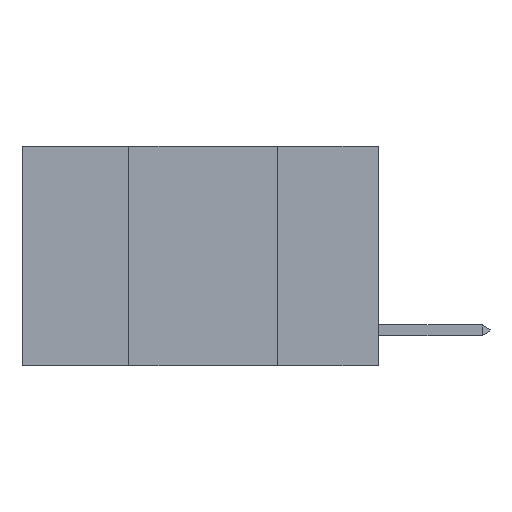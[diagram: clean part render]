
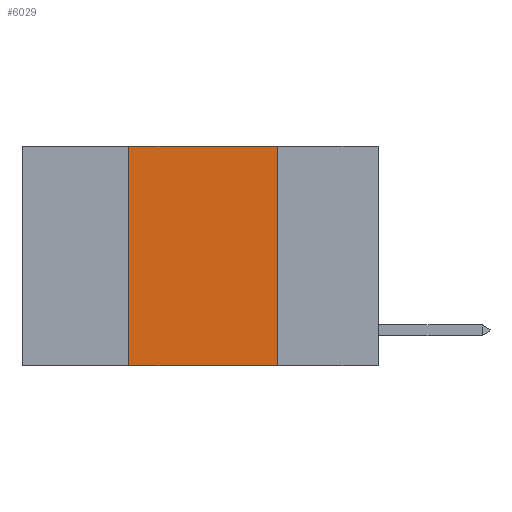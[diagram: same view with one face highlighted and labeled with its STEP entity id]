
A CAD part, left-side view. The second image highlights one B-rep face of the part: STEP entity #6029.
In plain terms, the highlighted planar face has unit normal (-1, 0, 0).
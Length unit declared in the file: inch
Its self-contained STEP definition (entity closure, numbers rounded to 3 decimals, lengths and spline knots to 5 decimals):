
#338 = CARTESIAN_POINT ( 'NONE',  ( 0., 0.6, 0. ) ) ;
#561 = EDGE_CURVE ( 'NONE', #802, #601, #5431, .T. ) ;
#601 = VERTEX_POINT ( 'NONE', #6798 ) ;
#706 = CARTESIAN_POINT ( 'NONE',  ( 0., 0.17, 0. ) ) ;
#802 = VERTEX_POINT ( 'NONE', #706 ) ;
#903 = DIRECTION ( 'NONE',  ( 0., -1., 0. ) ) ;
#1190 = ORIENTED_EDGE ( 'NONE', *, *, #10786, .F. ) ;
#1215 = VECTOR ( 'NONE', #3394, 39.37008 ) ;
#1487 = ORIENTED_EDGE ( 'NONE', *, *, #1878, .F. ) ;
#1836 = DIRECTION ( 'NONE',  ( 0., -1., 0. ) ) ;
#1878 = EDGE_CURVE ( 'NONE', #6333, #6514, #3742, .T. ) ;
#1903 = AXIS2_PLACEMENT_3D ( 'NONE', #338, #2266, #8986 ) ;
#2266 = DIRECTION ( 'NONE',  ( 1., 0., 0. ) ) ;
#3018 = DIRECTION ( 'NONE',  ( 0., 0., -1. ) ) ;
#3394 = DIRECTION ( 'NONE',  ( 0., 0., 1. ) ) ;
#3645 = CARTESIAN_POINT ( 'NONE',  ( 0., 0.42, 0. ) ) ;
#3742 = LINE ( 'NONE', #3645, #1215 ) ;
#4032 = ORIENTED_EDGE ( 'NONE', *, *, #10774, .T. ) ;
#4121 = CARTESIAN_POINT ( 'NONE',  ( 0., 0.42, -0.37 ) ) ;
#4162 = PLANE ( 'NONE',  #1903 ) ;
#4350 = VECTOR ( 'NONE', #903, 39.37008 ) ;
#5431 = LINE ( 'NONE', #8422, #7757 ) ;
#6015 = EDGE_LOOP ( 'NONE', ( #10958, #1190, #1487, #4032 ) ) ;
#6029 = ADVANCED_FACE ( 'NONE', ( #8960 ), #4162, .F. ) ;
#6333 = VERTEX_POINT ( 'NONE', #4121 ) ;
#6514 = VERTEX_POINT ( 'NONE', #11135 ) ;
#6798 = CARTESIAN_POINT ( 'NONE',  ( 0., 0.17, -0.37 ) ) ;
#7330 = LINE ( 'NONE', #12166, #4350 ) ;
#7757 = VECTOR ( 'NONE', #3018, 39.37008 ) ;
#8422 = CARTESIAN_POINT ( 'NONE',  ( 0., 0.17, 0. ) ) ;
#8960 = FACE_OUTER_BOUND ( 'NONE', #6015, .T. ) ;
#8986 = DIRECTION ( 'NONE',  ( 0., 0., -1. ) ) ;
#9433 = VECTOR ( 'NONE', #1836, 39.37008 ) ;
#9472 = CARTESIAN_POINT ( 'NONE',  ( 0., 0.6, -0.37 ) ) ;
#10774 = EDGE_CURVE ( 'NONE', #6333, #601, #11806, .T. ) ;
#10786 = EDGE_CURVE ( 'NONE', #6514, #802, #7330, .T. ) ;
#10958 = ORIENTED_EDGE ( 'NONE', *, *, #561, .F. ) ;
#11135 = CARTESIAN_POINT ( 'NONE',  ( 0., 0.42, 0. ) ) ;
#11806 = LINE ( 'NONE', #9472, #9433 ) ;
#12166 = CARTESIAN_POINT ( 'NONE',  ( 0., 0.6, 0. ) ) ;
